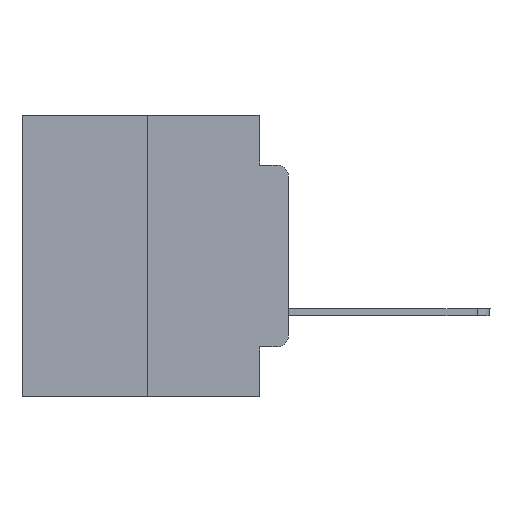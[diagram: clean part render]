
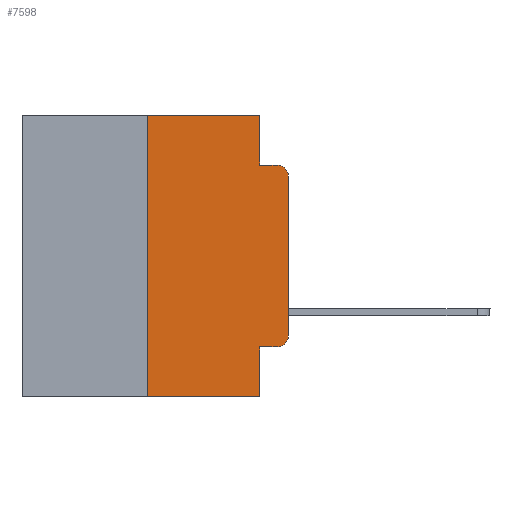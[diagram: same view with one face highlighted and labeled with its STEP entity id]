
A CAD part, left-side view. The second image highlights one B-rep face of the part: STEP entity #7598.
In plain terms, the highlighted planar face has unit normal (-1, 0, 0).
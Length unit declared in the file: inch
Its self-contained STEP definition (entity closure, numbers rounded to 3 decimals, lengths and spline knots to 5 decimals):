
#732 = ORIENTED_EDGE ( 'NONE', *, *, #23413, .T. ) ;
#1392 = VECTOR ( 'NONE', #25278, 39.37008 ) ;
#1588 = CARTESIAN_POINT ( 'NONE',  ( 0., 0., 0. ) ) ;
#1772 = EDGE_CURVE ( 'NONE', #14458, #7536, #18691, .T. ) ;
#2187 = EDGE_LOOP ( 'NONE', ( #732, #21492, #23123, #5858, #11702, #2411, #26525, #13728, #16920, #21029 ) ) ;
#2411 = ORIENTED_EDGE ( 'NONE', *, *, #4949, .F. ) ;
#2520 = CARTESIAN_POINT ( 'NONE',  ( 0., 0.25, 0. ) ) ;
#2523 = CARTESIAN_POINT ( 'NONE',  ( 0., 0.051, -0.0885 ) ) ;
#2567 = CARTESIAN_POINT ( 'NONE',  ( 0., 0.051, -0.5 ) ) ;
#2690 = VERTEX_POINT ( 'NONE', #2567 ) ;
#2901 = CARTESIAN_POINT ( 'NONE',  ( 0., 0.051, 0. ) ) ;
#3535 = CARTESIAN_POINT ( 'NONE',  ( 0., 0.051, 0. ) ) ;
#4149 = DIRECTION ( 'NONE',  ( 0., 0., 1. ) ) ;
#4458 = CARTESIAN_POINT ( 'NONE',  ( 0., 0., -0.1085 ) ) ;
#4825 = DIRECTION ( 'NONE',  ( 0., -1., 0. ) ) ;
#4949 = EDGE_CURVE ( 'NONE', #22644, #18541, #8388, .T. ) ;
#5116 = LINE ( 'NONE', #9067, #6739 ) ;
#5176 = CARTESIAN_POINT ( 'NONE',  ( 0., 0.02, -0.3915 ) ) ;
#5708 = DIRECTION ( 'NONE',  ( 0., -1., 0. ) ) ;
#5816 = CARTESIAN_POINT ( 'NONE',  ( 0., 0.02, -0.1085 ) ) ;
#5858 = ORIENTED_EDGE ( 'NONE', *, *, #1772, .F. ) ;
#5986 = VERTEX_POINT ( 'NONE', #22084 ) ;
#6453 = CARTESIAN_POINT ( 'NONE',  ( 0., 0.25, -0.5 ) ) ;
#6710 = VERTEX_POINT ( 'NONE', #24766 ) ;
#6739 = VECTOR ( 'NONE', #8944, 39.37008 ) ;
#7536 = VERTEX_POINT ( 'NONE', #15139 ) ;
#7598 = ADVANCED_FACE ( 'NONE', ( #22415 ), #11355, .F. ) ;
#7997 = DIRECTION ( 'NONE',  ( -1., 0., 0. ) ) ;
#8388 = LINE ( 'NONE', #2520, #15372 ) ;
#8592 = LINE ( 'NONE', #12672, #1392 ) ;
#8780 = EDGE_CURVE ( 'NONE', #7536, #12529, #12991, .T. ) ;
#8944 = DIRECTION ( 'NONE',  ( 0., -1., 0. ) ) ;
#9067 = CARTESIAN_POINT ( 'NONE',  ( 0., 0.051, -0.4115 ) ) ;
#9123 = DIRECTION ( 'NONE',  ( -1., 0., 0. ) ) ;
#9820 = CARTESIAN_POINT ( 'NONE',  ( 0., 0.473, 0. ) ) ;
#10772 = DIRECTION ( 'NONE',  ( 0., 0., -1. ) ) ;
#10834 = DIRECTION ( 'NONE',  ( 0., 0., -1. ) ) ;
#10843 = AXIS2_PLACEMENT_3D ( 'NONE', #5176, #9123, #10772 ) ;
#11201 = CARTESIAN_POINT ( 'NONE',  ( 0., 0., -0.3915 ) ) ;
#11355 = PLANE ( 'NONE',  #18978 ) ;
#11702 = ORIENTED_EDGE ( 'NONE', *, *, #12926, .F. ) ;
#11708 = CIRCLE ( 'NONE', #10843, 0.02 ) ;
#11799 = VECTOR ( 'NONE', #4825, 39.37008 ) ;
#11970 = CARTESIAN_POINT ( 'NONE',  ( 0., 0.25, 0. ) ) ;
#12025 = EDGE_CURVE ( 'NONE', #22644, #2690, #24292, .T. ) ;
#12086 = VERTEX_POINT ( 'NONE', #4458 ) ;
#12172 = CIRCLE ( 'NONE', #20392, 0.02 ) ;
#12529 = VERTEX_POINT ( 'NONE', #21234 ) ;
#12672 = CARTESIAN_POINT ( 'NONE',  ( 0., 0.473, 0. ) ) ;
#12926 = EDGE_CURVE ( 'NONE', #18541, #14458, #8592, .T. ) ;
#12991 = LINE ( 'NONE', #2523, #11799 ) ;
#13728 = ORIENTED_EDGE ( 'NONE', *, *, #21065, .F. ) ;
#14458 = VERTEX_POINT ( 'NONE', #3535 ) ;
#15139 = CARTESIAN_POINT ( 'NONE',  ( 0., 0.051, -0.0885 ) ) ;
#15372 = VECTOR ( 'NONE', #4149, 39.37008 ) ;
#16888 = VERTEX_POINT ( 'NONE', #11201 ) ;
#16920 = ORIENTED_EDGE ( 'NONE', *, *, #26744, .T. ) ;
#17572 = DIRECTION ( 'NONE',  ( 1., 0., 0. ) ) ;
#17839 = VECTOR ( 'NONE', #5708, 39.37008 ) ;
#18077 = DIRECTION ( 'NONE',  ( 0., 0., -1. ) ) ;
#18541 = VERTEX_POINT ( 'NONE', #11970 ) ;
#18691 = LINE ( 'NONE', #22765, #23708 ) ;
#18978 = AXIS2_PLACEMENT_3D ( 'NONE', #9820, #17572, #18077 ) ;
#20128 = EDGE_CURVE ( 'NONE', #5986, #16888, #11708, .T. ) ;
#20392 = AXIS2_PLACEMENT_3D ( 'NONE', #5816, #7997, #24544 ) ;
#20924 = EDGE_CURVE ( 'NONE', #12086, #12529, #12172, .T. ) ;
#21029 = ORIENTED_EDGE ( 'NONE', *, *, #20128, .T. ) ;
#21065 = EDGE_CURVE ( 'NONE', #6710, #2690, #21144, .T. ) ;
#21144 = LINE ( 'NONE', #2901, #25603 ) ;
#21234 = CARTESIAN_POINT ( 'NONE',  ( 0., 0.02, -0.0885 ) ) ;
#21492 = ORIENTED_EDGE ( 'NONE', *, *, #20924, .T. ) ;
#21640 = DIRECTION ( 'NONE',  ( 0., 0., -1. ) ) ;
#21959 = DIRECTION ( 'NONE',  ( 0., 0., 1. ) ) ;
#22084 = CARTESIAN_POINT ( 'NONE',  ( 0., 0.02, -0.4115 ) ) ;
#22170 = VECTOR ( 'NONE', #21959, 39.37008 ) ;
#22415 = FACE_OUTER_BOUND ( 'NONE', #2187, .T. ) ;
#22644 = VERTEX_POINT ( 'NONE', #6453 ) ;
#22765 = CARTESIAN_POINT ( 'NONE',  ( 0., 0.051, 0. ) ) ;
#23123 = ORIENTED_EDGE ( 'NONE', *, *, #8780, .F. ) ;
#23413 = EDGE_CURVE ( 'NONE', #16888, #12086, #23872, .T. ) ;
#23708 = VECTOR ( 'NONE', #10834, 39.37008 ) ;
#23872 = LINE ( 'NONE', #1588, #22170 ) ;
#24038 = CARTESIAN_POINT ( 'NONE',  ( 0., 0.473, -0.5 ) ) ;
#24292 = LINE ( 'NONE', #24038, #17839 ) ;
#24544 = DIRECTION ( 'NONE',  ( 0., 0., -1. ) ) ;
#24766 = CARTESIAN_POINT ( 'NONE',  ( 0., 0.051, -0.4115 ) ) ;
#25278 = DIRECTION ( 'NONE',  ( 0., -1., 0. ) ) ;
#25603 = VECTOR ( 'NONE', #21640, 39.37008 ) ;
#26525 = ORIENTED_EDGE ( 'NONE', *, *, #12025, .T. ) ;
#26744 = EDGE_CURVE ( 'NONE', #6710, #5986, #5116, .T. ) ;
